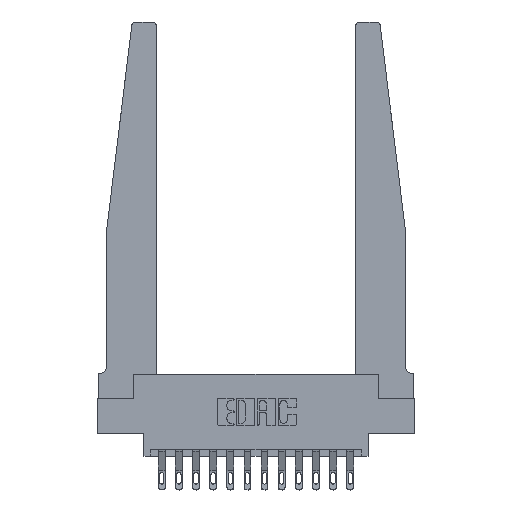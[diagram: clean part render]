
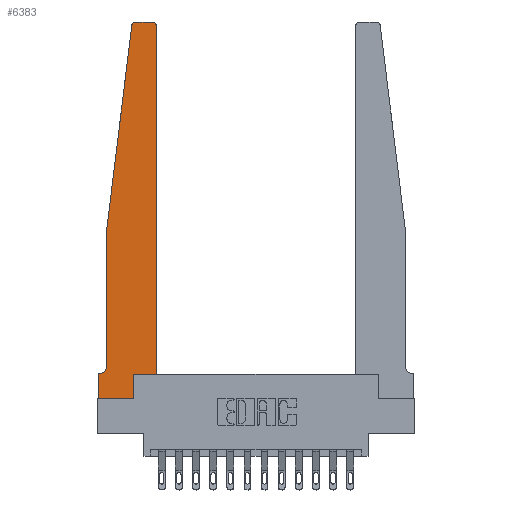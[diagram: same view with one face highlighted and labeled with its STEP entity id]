
A CAD part, top view. The second image highlights one B-rep face of the part: STEP entity #6383.
In plain terms, the highlighted planar face has unit normal (0, 0, 1).
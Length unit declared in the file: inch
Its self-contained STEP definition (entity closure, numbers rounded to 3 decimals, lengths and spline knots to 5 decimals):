
#66 = CARTESIAN_POINT ( 'NONE',  ( 0.25, 2.75, 0.37 ) ) ;
#185 = CIRCLE ( 'NONE', #4196, 0.05 ) ;
#271 = VECTOR ( 'NONE', #16545, 39.37008 ) ;
#321 = DIRECTION ( 'NONE',  ( 0., -1., 0. ) ) ;
#325 = DIRECTION ( 'NONE',  ( -1., 0., 0. ) ) ;
#353 = CARTESIAN_POINT ( 'NONE',  ( 0.015, 0.1875, 0.37 ) ) ;
#389 = LINE ( 'NONE', #3257, #271 ) ;
#462 = VERTEX_POINT ( 'NONE', #783 ) ;
#510 = ORIENTED_EDGE ( 'NONE', *, *, #1689, .T. ) ;
#783 = CARTESIAN_POINT ( 'NONE',  ( 0.065, 0.2375, 0.37 ) ) ;
#819 = EDGE_CURVE ( 'NONE', #16152, #895, #7102, .T. ) ;
#895 = VERTEX_POINT ( 'NONE', #6131 ) ;
#1082 = CARTESIAN_POINT ( 'NONE',  ( 0., 0., 0.37 ) ) ;
#1529 = DIRECTION ( 'NONE',  ( 1., 0., 0. ) ) ;
#1653 = VERTEX_POINT ( 'NONE', #12760 ) ;
#1664 = CARTESIAN_POINT ( 'NONE',  ( 0.2605, 0.18, 0.37 ) ) ;
#1689 = EDGE_CURVE ( 'NONE', #1653, #15498, #7477, .T. ) ;
#1727 = DIRECTION ( 'NONE',  ( 0., 1., 0. ) ) ;
#1911 = DIRECTION ( 'NONE',  ( 0., -1., 0. ) ) ;
#2092 = CARTESIAN_POINT ( 'NONE',  ( 0.065, 1.25, 0.37 ) ) ;
#2234 = EDGE_CURVE ( 'NONE', #462, #16152, #185, .T. ) ;
#2447 = AXIS2_PLACEMENT_3D ( 'NONE', #14877, #12947, #11619 ) ;
#2469 = CARTESIAN_POINT ( 'NONE',  ( 0.395, 2.72, 0.37 ) ) ;
#2616 = EDGE_CURVE ( 'NONE', #895, #11806, #7168, .T. ) ;
#2702 = VECTOR ( 'NONE', #14681, 39.37008 ) ;
#2962 = VECTOR ( 'NONE', #12560, 39.37008 ) ;
#3078 = CARTESIAN_POINT ( 'NONE',  ( 0.27653, 2.75, 0.37 ) ) ;
#3208 = VERTEX_POINT ( 'NONE', #13573 ) ;
#3257 = CARTESIAN_POINT ( 'NONE',  ( 0.425, 0.18, 0.37 ) ) ;
#3259 = VECTOR ( 'NONE', #12848, 39.37008 ) ;
#4174 = CIRCLE ( 'NONE', #2447, 0.03 ) ;
#4196 = AXIS2_PLACEMENT_3D ( 'NONE', #17345, #13363, #9305 ) ;
#4202 = EDGE_CURVE ( 'NONE', #16065, #14162, #5787, .T. ) ;
#4597 = CARTESIAN_POINT ( 'NONE',  ( 0., 0., 0.37 ) ) ;
#4615 = EDGE_LOOP ( 'NONE', ( #14281, #14460, #510, #17127, #16301, #11617, #5783, #14915, #7685, #15889, #12711, #9236 ) ) ;
#4637 = EDGE_CURVE ( 'NONE', #5306, #9168, #389, .T. ) ;
#4716 = VERTEX_POINT ( 'NONE', #7610 ) ;
#5306 = VERTEX_POINT ( 'NONE', #6864 ) ;
#5783 = ORIENTED_EDGE ( 'NONE', *, *, #2616, .T. ) ;
#5787 = LINE ( 'NONE', #66, #6791 ) ;
#6131 = CARTESIAN_POINT ( 'NONE',  ( 0., 0.1875, 0.37 ) ) ;
#6324 = CARTESIAN_POINT ( 'NONE',  ( 0.065, 1.25, 0.37 ) ) ;
#6383 = ADVANCED_FACE ( 'NONE', ( #6605 ), #16081, .T. ) ;
#6475 = DIRECTION ( 'NONE',  ( 1., 0., 0. ) ) ;
#6605 = FACE_OUTER_BOUND ( 'NONE', #4615, .T. ) ;
#6791 = VECTOR ( 'NONE', #13473, 39.37008 ) ;
#6864 = CARTESIAN_POINT ( 'NONE',  ( 0.2605, 0.18, 0.37 ) ) ;
#7009 = LINE ( 'NONE', #1664, #2962 ) ;
#7099 = LINE ( 'NONE', #12473, #13350 ) ;
#7102 = LINE ( 'NONE', #8235, #13117 ) ;
#7168 = LINE ( 'NONE', #4597, #14361 ) ;
#7428 = LINE ( 'NONE', #12804, #17106 ) ;
#7477 = LINE ( 'NONE', #6324, #3259 ) ;
#7610 = CARTESIAN_POINT ( 'NONE',  ( 0.2605, 0., 0.37 ) ) ;
#7685 = ORIENTED_EDGE ( 'NONE', *, *, #13849, .T. ) ;
#7939 = AXIS2_PLACEMENT_3D ( 'NONE', #13668, #8267, #1529 ) ;
#7970 = EDGE_CURVE ( 'NONE', #15498, #462, #7099, .T. ) ;
#8235 = CARTESIAN_POINT ( 'NONE',  ( 0.065, 0.1875, 0.37 ) ) ;
#8267 = DIRECTION ( 'NONE',  ( 0., 0., 1. ) ) ;
#8326 = CARTESIAN_POINT ( 'NONE',  ( 0.425, 0.18, 0.37 ) ) ;
#9168 = VERTEX_POINT ( 'NONE', #8326 ) ;
#9236 = ORIENTED_EDGE ( 'NONE', *, *, #15104, .T. ) ;
#9305 = DIRECTION ( 'NONE',  ( -1., 0., 0. ) ) ;
#9830 = EDGE_CURVE ( 'NONE', #9168, #3208, #7428, .T. ) ;
#10599 = LINE ( 'NONE', #16016, #2702 ) ;
#11617 = ORIENTED_EDGE ( 'NONE', *, *, #819, .T. ) ;
#11619 = DIRECTION ( 'NONE',  ( 1., 0., 0. ) ) ;
#11806 = VERTEX_POINT ( 'NONE', #1082 ) ;
#12473 = CARTESIAN_POINT ( 'NONE',  ( 0.065, 1.25, 0.37 ) ) ;
#12560 = DIRECTION ( 'NONE',  ( 0., 1., 0. ) ) ;
#12603 = CIRCLE ( 'NONE', #16847, 0.03 ) ;
#12711 = ORIENTED_EDGE ( 'NONE', *, *, #9830, .T. ) ;
#12760 = CARTESIAN_POINT ( 'NONE',  ( 0.24675, 2.72367, 0.37 ) ) ;
#12804 = CARTESIAN_POINT ( 'NONE',  ( 0.425, 0.18, 0.37 ) ) ;
#12848 = DIRECTION ( 'NONE',  ( -0.122, -0.992, 0. ) ) ;
#12947 = DIRECTION ( 'NONE',  ( 0., 0., 1. ) ) ;
#13117 = VECTOR ( 'NONE', #325, 39.37008 ) ;
#13350 = VECTOR ( 'NONE', #321, 39.37008 ) ;
#13363 = DIRECTION ( 'NONE',  ( 0., 0., -1. ) ) ;
#13473 = DIRECTION ( 'NONE',  ( -1., 0., 0. ) ) ;
#13573 = CARTESIAN_POINT ( 'NONE',  ( 0.425, 2.72, 0.37 ) ) ;
#13668 = CARTESIAN_POINT ( 'NONE',  ( 0., 0.1875, 0.37 ) ) ;
#13849 = EDGE_CURVE ( 'NONE', #4716, #5306, #7009, .T. ) ;
#14162 = VERTEX_POINT ( 'NONE', #3078 ) ;
#14281 = ORIENTED_EDGE ( 'NONE', *, *, #4202, .T. ) ;
#14361 = VECTOR ( 'NONE', #1911, 39.37008 ) ;
#14460 = ORIENTED_EDGE ( 'NONE', *, *, #16282, .T. ) ;
#14610 = DIRECTION ( 'NONE',  ( 0., 0., 1. ) ) ;
#14681 = DIRECTION ( 'NONE',  ( 1., 0., 0. ) ) ;
#14877 = CARTESIAN_POINT ( 'NONE',  ( 0.27653, 2.72, 0.37 ) ) ;
#14915 = ORIENTED_EDGE ( 'NONE', *, *, #16933, .T. ) ;
#15104 = EDGE_CURVE ( 'NONE', #3208, #16065, #12603, .T. ) ;
#15498 = VERTEX_POINT ( 'NONE', #2092 ) ;
#15889 = ORIENTED_EDGE ( 'NONE', *, *, #4637, .T. ) ;
#16016 = CARTESIAN_POINT ( 'NONE',  ( 0., 0., 0.37 ) ) ;
#16065 = VERTEX_POINT ( 'NONE', #16248 ) ;
#16081 = PLANE ( 'NONE',  #7939 ) ;
#16152 = VERTEX_POINT ( 'NONE', #353 ) ;
#16248 = CARTESIAN_POINT ( 'NONE',  ( 0.395, 2.75, 0.37 ) ) ;
#16282 = EDGE_CURVE ( 'NONE', #14162, #1653, #4174, .T. ) ;
#16301 = ORIENTED_EDGE ( 'NONE', *, *, #2234, .T. ) ;
#16545 = DIRECTION ( 'NONE',  ( 1., 0., 0. ) ) ;
#16847 = AXIS2_PLACEMENT_3D ( 'NONE', #2469, #14610, #6475 ) ;
#16933 = EDGE_CURVE ( 'NONE', #11806, #4716, #10599, .T. ) ;
#17106 = VECTOR ( 'NONE', #1727, 39.37008 ) ;
#17127 = ORIENTED_EDGE ( 'NONE', *, *, #7970, .T. ) ;
#17345 = CARTESIAN_POINT ( 'NONE',  ( 0.015, 0.2375, 0.37 ) ) ;
